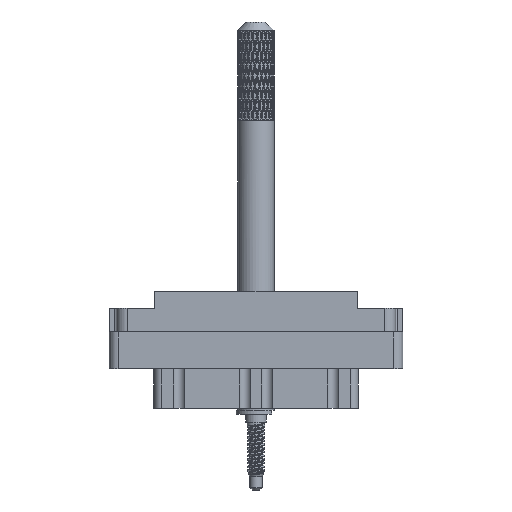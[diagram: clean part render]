
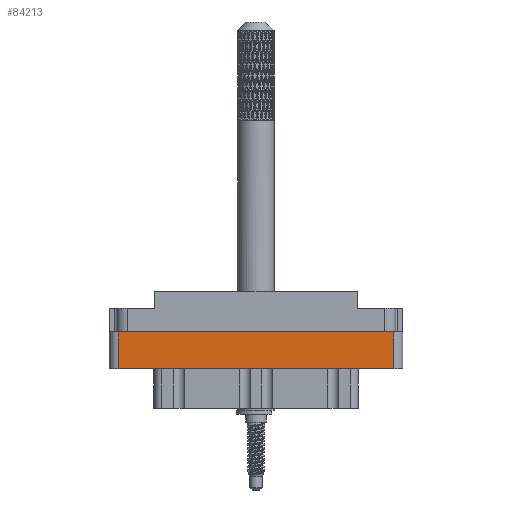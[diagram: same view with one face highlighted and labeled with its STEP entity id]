
A CAD part, front view. The second image highlights one B-rep face of the part: STEP entity #84213.
In plain terms, the highlighted planar face has unit normal (0, -1, 0).
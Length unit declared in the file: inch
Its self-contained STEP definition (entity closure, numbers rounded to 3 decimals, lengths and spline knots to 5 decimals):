
#3230 = LINE ( 'NONE', #33570, #79378 ) ;
#6723 = PLANE ( 'NONE',  #42264 ) ;
#9124 = VERTEX_POINT ( 'NONE', #24936 ) ;
#9129 = CARTESIAN_POINT ( 'NONE',  ( -0.938, -0.438, -0.277 ) ) ;
#15793 = VECTOR ( 'NONE', #85822, 39.37008 ) ;
#20415 = CARTESIAN_POINT ( 'NONE',  ( -0.938, -0.438, -0.529 ) ) ;
#22388 = EDGE_CURVE ( 'NONE', #9124, #72525, #3230, .T. ) ;
#22793 = VERTEX_POINT ( 'NONE', #9129 ) ;
#24781 = VECTOR ( 'NONE', #58603, 39.37008 ) ;
#24936 = CARTESIAN_POINT ( 'NONE',  ( 0.938, -0.438, -0.529 ) ) ;
#33570 = CARTESIAN_POINT ( 'NONE',  ( 0.938, -0.438, -0.798 ) ) ;
#33749 = CARTESIAN_POINT ( 'NONE',  ( 0.938, -0.438, -0.529 ) ) ;
#35215 = VECTOR ( 'NONE', #62580, 39.37008 ) ;
#38008 = DIRECTION ( 'NONE',  ( 0., 0., -1. ) ) ;
#39196 = EDGE_CURVE ( 'NONE', #9124, #81209, #70046, .T. ) ;
#42264 = AXIS2_PLACEMENT_3D ( 'NONE', #67330, #91211, #38008 ) ;
#44189 = CARTESIAN_POINT ( 'NONE',  ( -0.938, -0.438, -0.798 ) ) ;
#45015 = EDGE_CURVE ( 'NONE', #22793, #72525, #47056, .T. ) ;
#47056 = LINE ( 'NONE', #55496, #15793 ) ;
#47533 = ORIENTED_EDGE ( 'NONE', *, *, #22388, .T. ) ;
#48968 = DIRECTION ( 'NONE',  ( 0., 0., 1. ) ) ;
#49307 = ORIENTED_EDGE ( 'NONE', *, *, #45015, .F. ) ;
#51662 = LINE ( 'NONE', #44189, #24781 ) ;
#51955 = FACE_OUTER_BOUND ( 'NONE', #52614, .T. ) ;
#52614 = EDGE_LOOP ( 'NONE', ( #90024, #80517, #47533, #49307 ) ) ;
#55496 = CARTESIAN_POINT ( 'NONE',  ( -1., -0.438, -0.277 ) ) ;
#58603 = DIRECTION ( 'NONE',  ( 0., 0., 1. ) ) ;
#62580 = DIRECTION ( 'NONE',  ( -1., 0., 0. ) ) ;
#64916 = EDGE_CURVE ( 'NONE', #81209, #22793, #51662, .T. ) ;
#67330 = CARTESIAN_POINT ( 'NONE',  ( -0.938, -0.438, -0.798 ) ) ;
#70046 = LINE ( 'NONE', #33749, #35215 ) ;
#72309 = CARTESIAN_POINT ( 'NONE',  ( 0.938, -0.438, -0.277 ) ) ;
#72525 = VERTEX_POINT ( 'NONE', #72309 ) ;
#79378 = VECTOR ( 'NONE', #48968, 39.37008 ) ;
#80517 = ORIENTED_EDGE ( 'NONE', *, *, #39196, .F. ) ;
#81209 = VERTEX_POINT ( 'NONE', #20415 ) ;
#84213 = ADVANCED_FACE ( 'NONE', ( #51955 ), #6723, .T. ) ;
#85822 = DIRECTION ( 'NONE',  ( 1., 0., 0. ) ) ;
#90024 = ORIENTED_EDGE ( 'NONE', *, *, #64916, .F. ) ;
#91211 = DIRECTION ( 'NONE',  ( 0., -1., 0. ) ) ;
